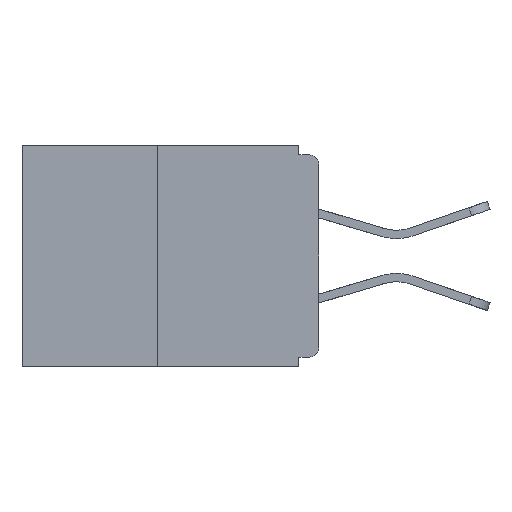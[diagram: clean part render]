
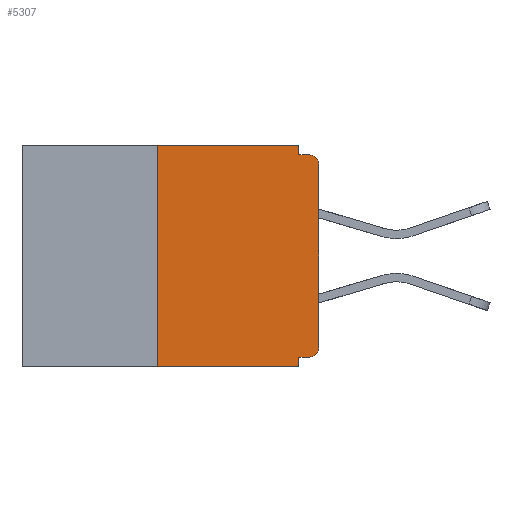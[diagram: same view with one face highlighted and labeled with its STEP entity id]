
A CAD part, left-side view. The second image highlights one B-rep face of the part: STEP entity #5307.
In plain terms, the highlighted planar face has unit normal (-1, 0, 0).
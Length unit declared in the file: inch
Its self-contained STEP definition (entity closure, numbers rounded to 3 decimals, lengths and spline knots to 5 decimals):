
#418 = VECTOR ( 'NONE', #12866, 39.37008 ) ;
#578 = CARTESIAN_POINT ( 'NONE',  ( 0., 0.031, -0.328 ) ) ;
#639 = EDGE_CURVE ( 'NONE', #2054, #3853, #1165, .T. ) ;
#649 = CIRCLE ( 'NONE', #10855, 0.015 ) ;
#721 = ORIENTED_EDGE ( 'NONE', *, *, #12210, .T. ) ;
#808 = EDGE_CURVE ( 'NONE', #1986, #12276, #8323, .T. ) ;
#963 = DIRECTION ( 'NONE',  ( 0., 0., -1. ) ) ;
#1037 = CARTESIAN_POINT ( 'NONE',  ( 0., 0., 0. ) ) ;
#1165 = LINE ( 'NONE', #8904, #6618 ) ;
#1371 = VERTEX_POINT ( 'NONE', #4357 ) ;
#1783 = ORIENTED_EDGE ( 'NONE', *, *, #3325, .F. ) ;
#1934 = ORIENTED_EDGE ( 'NONE', *, *, #12263, .F. ) ;
#1986 = VERTEX_POINT ( 'NONE', #578 ) ;
#2018 = VECTOR ( 'NONE', #11669, 39.37008 ) ;
#2054 = VERTEX_POINT ( 'NONE', #8899 ) ;
#2583 = ORIENTED_EDGE ( 'NONE', *, *, #6332, .T. ) ;
#2603 = AXIS2_PLACEMENT_3D ( 'NONE', #10763, #3992, #963 ) ;
#2715 = PLANE ( 'NONE',  #2603 ) ;
#2806 = ORIENTED_EDGE ( 'NONE', *, *, #9355, .T. ) ;
#2815 = VERTEX_POINT ( 'NONE', #11579 ) ;
#3026 = DIRECTION ( 'NONE',  ( 0., 0., 1. ) ) ;
#3265 = VERTEX_POINT ( 'NONE', #3878 ) ;
#3325 = EDGE_CURVE ( 'NONE', #3853, #8453, #7458, .T. ) ;
#3687 = DIRECTION ( 'NONE',  ( -1., 0., 0. ) ) ;
#3794 = DIRECTION ( 'NONE',  ( 0., 0., -1. ) ) ;
#3843 = LINE ( 'NONE', #12239, #11808 ) ;
#3853 = VERTEX_POINT ( 'NONE', #10335 ) ;
#3878 = CARTESIAN_POINT ( 'NONE',  ( 0., 0., -0.313 ) ) ;
#3897 = LINE ( 'NONE', #4689, #2018 ) ;
#3929 = LINE ( 'NONE', #1037, #12516 ) ;
#3950 = VERTEX_POINT ( 'NONE', #8138 ) ;
#3992 = DIRECTION ( 'NONE',  ( 1., 0., 0. ) ) ;
#4130 = DIRECTION ( 'NONE',  ( -1., 0., 0. ) ) ;
#4357 = CARTESIAN_POINT ( 'NONE',  ( 0., 0.015, -0.015 ) ) ;
#4529 = EDGE_CURVE ( 'NONE', #3950, #1371, #649, .T. ) ;
#4547 = EDGE_CURVE ( 'NONE', #7199, #1986, #3897, .T. ) ;
#4631 = ORIENTED_EDGE ( 'NONE', *, *, #808, .F. ) ;
#4689 = CARTESIAN_POINT ( 'NONE',  ( 0., 0., -0.328 ) ) ;
#4866 = ORIENTED_EDGE ( 'NONE', *, *, #4547, .F. ) ;
#4984 = DIRECTION ( 'NONE',  ( 0., -1., 0. ) ) ;
#5000 = EDGE_LOOP ( 'NONE', ( #12660, #5573, #2806, #4631, #4866, #721, #2583, #7608, #1934, #1783 ) ) ;
#5126 = DIRECTION ( 'NONE',  ( 0., -1., 0. ) ) ;
#5173 = CARTESIAN_POINT ( 'NONE',  ( 0., 0.031, -0.015 ) ) ;
#5280 = CARTESIAN_POINT ( 'NONE',  ( 0., 0.031, -0.343 ) ) ;
#5307 = ADVANCED_FACE ( 'NONE', ( #11770 ), #2715, .F. ) ;
#5558 = CIRCLE ( 'NONE', #7889, 0.015 ) ;
#5573 = ORIENTED_EDGE ( 'NONE', *, *, #12816, .F. ) ;
#5825 = VECTOR ( 'NONE', #10259, 39.37008 ) ;
#6332 = EDGE_CURVE ( 'NONE', #3265, #3950, #3929, .T. ) ;
#6618 = VECTOR ( 'NONE', #4984, 39.37008 ) ;
#6825 = CARTESIAN_POINT ( 'NONE',  ( 0., 0.015, -0.328 ) ) ;
#7030 = CARTESIAN_POINT ( 'NONE',  ( 0., 0.015, -0.313 ) ) ;
#7096 = VECTOR ( 'NONE', #5126, 39.37008 ) ;
#7134 = VECTOR ( 'NONE', #3794, 39.37008 ) ;
#7199 = VERTEX_POINT ( 'NONE', #6825 ) ;
#7458 = LINE ( 'NONE', #9828, #7134 ) ;
#7608 = ORIENTED_EDGE ( 'NONE', *, *, #4529, .T. ) ;
#7889 = AXIS2_PLACEMENT_3D ( 'NONE', #7030, #4130, #10986 ) ;
#8138 = CARTESIAN_POINT ( 'NONE',  ( 0., 0., -0.03 ) ) ;
#8323 = LINE ( 'NONE', #5280, #5825 ) ;
#8453 = VERTEX_POINT ( 'NONE', #5173 ) ;
#8899 = CARTESIAN_POINT ( 'NONE',  ( 0., 0.25, 0. ) ) ;
#8904 = CARTESIAN_POINT ( 'NONE',  ( 0., 0.46, 0. ) ) ;
#9355 = EDGE_CURVE ( 'NONE', #2815, #12276, #3843, .T. ) ;
#9634 = CARTESIAN_POINT ( 'NONE',  ( 0., 0.015, -0.03 ) ) ;
#9754 = CARTESIAN_POINT ( 'NONE',  ( 0., 0.25, 0. ) ) ;
#9828 = CARTESIAN_POINT ( 'NONE',  ( 0., 0.031, 0. ) ) ;
#9999 = CARTESIAN_POINT ( 'NONE',  ( 0., 0.031, -0.343 ) ) ;
#10259 = DIRECTION ( 'NONE',  ( 0., 0., -1. ) ) ;
#10335 = CARTESIAN_POINT ( 'NONE',  ( 0., 0.031, 0. ) ) ;
#10591 = DIRECTION ( 'NONE',  ( 0., -1., 0. ) ) ;
#10664 = DIRECTION ( 'NONE',  ( 0., 0., -1. ) ) ;
#10763 = CARTESIAN_POINT ( 'NONE',  ( 0., 0.46, 0. ) ) ;
#10855 = AXIS2_PLACEMENT_3D ( 'NONE', #9634, #3687, #10664 ) ;
#10986 = DIRECTION ( 'NONE',  ( 0., 0., -1. ) ) ;
#11107 = CARTESIAN_POINT ( 'NONE',  ( 0., 0., -0.015 ) ) ;
#11150 = LINE ( 'NONE', #9754, #418 ) ;
#11579 = CARTESIAN_POINT ( 'NONE',  ( 0., 0.25, -0.343 ) ) ;
#11669 = DIRECTION ( 'NONE',  ( 0., 1., 0. ) ) ;
#11770 = FACE_OUTER_BOUND ( 'NONE', #5000, .T. ) ;
#11808 = VECTOR ( 'NONE', #10591, 39.37008 ) ;
#12108 = LINE ( 'NONE', #11107, #7096 ) ;
#12210 = EDGE_CURVE ( 'NONE', #7199, #3265, #5558, .T. ) ;
#12239 = CARTESIAN_POINT ( 'NONE',  ( 0., 0.46, -0.343 ) ) ;
#12263 = EDGE_CURVE ( 'NONE', #8453, #1371, #12108, .T. ) ;
#12276 = VERTEX_POINT ( 'NONE', #9999 ) ;
#12516 = VECTOR ( 'NONE', #3026, 39.37008 ) ;
#12660 = ORIENTED_EDGE ( 'NONE', *, *, #639, .F. ) ;
#12816 = EDGE_CURVE ( 'NONE', #2815, #2054, #11150, .T. ) ;
#12866 = DIRECTION ( 'NONE',  ( 0., 0., 1. ) ) ;
